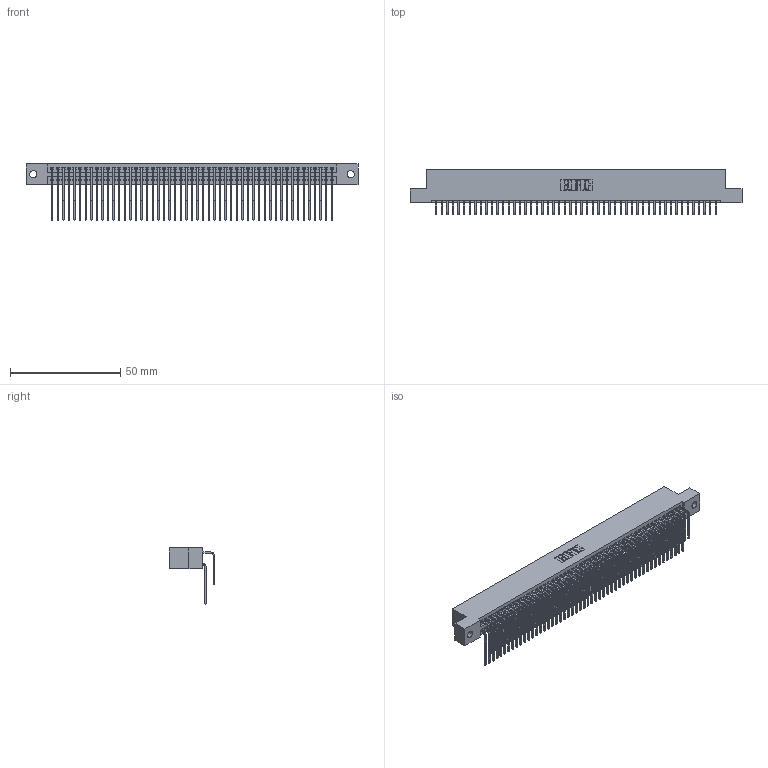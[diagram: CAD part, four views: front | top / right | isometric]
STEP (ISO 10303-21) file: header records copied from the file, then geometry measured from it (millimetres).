
FILE_DESCRIPTION (( 'STEP AP203' ), '1' );
FILE_NAME ('345-102-559-202.STEP', '2019-11-03T09:26:38', ( '' ), ( '' ), 'SwSTEP 2.0', 'SolidWorks 2016', '' );
FILE_SCHEMA (( 'CONFIG_CONTROL_DESIGN' ));
Length unit declared in the file: inch
Products named in the file (4): 345-292-001_559 Tail - 2; 345-102-559-202; 345-292-001_558 559 Tail - 1; 345 Part_Flush Mounting Lugs - 0.128 Dia
Assembly tree (103 placements, depth 2):
  345-102-559-202
    345 Part_Flush Mounting Lugs - 0.128 Dia
    345-292-001_558 559 Tail - 1  x51
    345-292-001_559 Tail - 2  x51
Bounding box: 150.75 x 20.56 x 25.53 mm (x, y, z)
Volume: 15279.2 mm3; surface area: 25253.7 mm2
Topology: 103 solids, 103 shells, 5430 faces, 16151 edges, 10630 vertices
Faces by surface type: plane 3650, cylinder 1780
Entity records: 40459 total; most frequent: CARTESIAN_POINT 6819, ORIENTED_EDGE 6702, DIRECTION 5975, EDGE_CURVE 3351, VECTOR 2975, LINE 2975, VERTEX_POINT 2230, AXIS2_PLACEMENT_3D 1500
